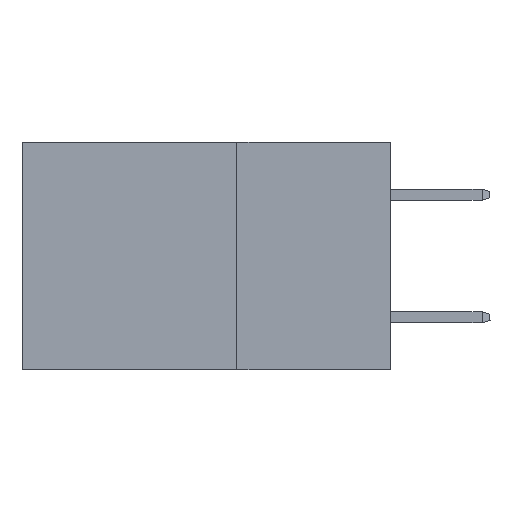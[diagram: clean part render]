
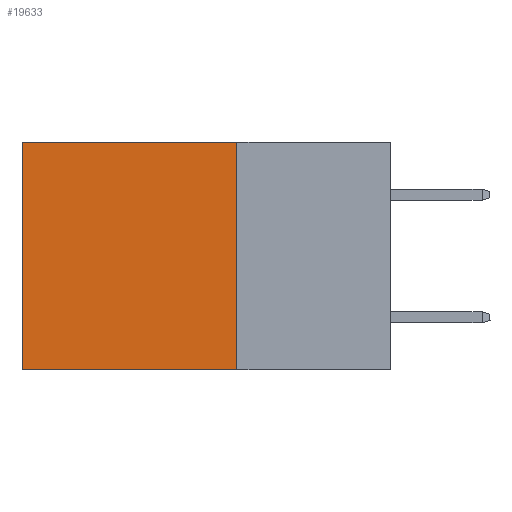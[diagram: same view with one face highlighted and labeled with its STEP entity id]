
A CAD part, left-side view. The second image highlights one B-rep face of the part: STEP entity #19633.
In plain terms, the highlighted planar face has unit normal (-1, 0, 0).
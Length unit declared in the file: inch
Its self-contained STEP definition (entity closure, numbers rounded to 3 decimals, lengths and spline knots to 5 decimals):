
#140 = CARTESIAN_POINT ( 'NONE',  ( 0.2875, 0.25, 0. ) ) ;
#1378 = CARTESIAN_POINT ( 'NONE',  ( 0.2875, 0.25, -0.37 ) ) ;
#2064 = CARTESIAN_POINT ( 'NONE',  ( 0.2875, 0.25, 0. ) ) ;
#2134 = VERTEX_POINT ( 'NONE', #6580 ) ;
#2252 = LINE ( 'NONE', #15097, #31841 ) ;
#2772 = EDGE_CURVE ( 'NONE', #35633, #2134, #17829, .T. ) ;
#3504 = ORIENTED_EDGE ( 'NONE', *, *, #4121, .T. ) ;
#4121 = EDGE_CURVE ( 'NONE', #35633, #14158, #2252, .T. ) ;
#4724 = VERTEX_POINT ( 'NONE', #8125 ) ;
#5948 = EDGE_LOOP ( 'NONE', ( #37358, #40906, #30566, #3504 ) ) ;
#6580 = CARTESIAN_POINT ( 'NONE',  ( 0.2875, 0.25, -0.37 ) ) ;
#7094 = EDGE_CURVE ( 'NONE', #2134, #4724, #13004, .T. ) ;
#7177 = AXIS2_PLACEMENT_3D ( 'NONE', #8513, #30518, #11330 ) ;
#8125 = CARTESIAN_POINT ( 'NONE',  ( 0.2875, 0.6, -0.37 ) ) ;
#8513 = CARTESIAN_POINT ( 'NONE',  ( 0.2875, 0.25, 0. ) ) ;
#10299 = VECTOR ( 'NONE', #29716, 39.37008 ) ;
#11330 = DIRECTION ( 'NONE',  ( 0., 0., -1. ) ) ;
#13004 = LINE ( 'NONE', #1378, #19044 ) ;
#13832 = CARTESIAN_POINT ( 'NONE',  ( 0.2875, 0.6, 0. ) ) ;
#14158 = VERTEX_POINT ( 'NONE', #15800 ) ;
#15097 = CARTESIAN_POINT ( 'NONE',  ( 0.2875, 0.25, 0. ) ) ;
#15800 = CARTESIAN_POINT ( 'NONE',  ( 0.2875, 0.6, 0. ) ) ;
#17829 = LINE ( 'NONE', #140, #10299 ) ;
#19044 = VECTOR ( 'NONE', #20302, 39.37008 ) ;
#19633 = ADVANCED_FACE ( 'NONE', ( #39610 ), #24231, .F. ) ;
#20302 = DIRECTION ( 'NONE',  ( 0., 1., 0. ) ) ;
#21299 = VECTOR ( 'NONE', #36662, 39.37008 ) ;
#24231 = PLANE ( 'NONE',  #7177 ) ;
#29716 = DIRECTION ( 'NONE',  ( 0., 0., -1. ) ) ;
#30307 = LINE ( 'NONE', #13832, #21299 ) ;
#30518 = DIRECTION ( 'NONE',  ( 1., 0., 0. ) ) ;
#30566 = ORIENTED_EDGE ( 'NONE', *, *, #2772, .F. ) ;
#31835 = EDGE_CURVE ( 'NONE', #14158, #4724, #30307, .T. ) ;
#31841 = VECTOR ( 'NONE', #34565, 39.37008 ) ;
#34565 = DIRECTION ( 'NONE',  ( 0., 1., 0. ) ) ;
#35633 = VERTEX_POINT ( 'NONE', #2064 ) ;
#36662 = DIRECTION ( 'NONE',  ( 0., 0., -1. ) ) ;
#37358 = ORIENTED_EDGE ( 'NONE', *, *, #31835, .T. ) ;
#39610 = FACE_OUTER_BOUND ( 'NONE', #5948, .T. ) ;
#40906 = ORIENTED_EDGE ( 'NONE', *, *, #7094, .F. ) ;
